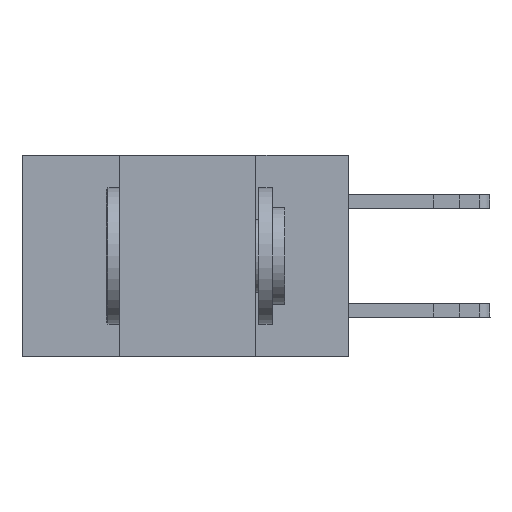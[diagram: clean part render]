
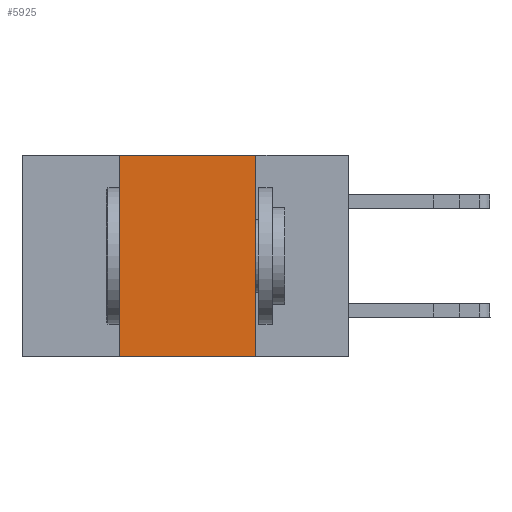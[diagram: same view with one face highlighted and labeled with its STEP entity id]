
A CAD part, left-side view. The second image highlights one B-rep face of the part: STEP entity #5925.
In plain terms, the highlighted planar face has unit normal (-1, 0, 0).
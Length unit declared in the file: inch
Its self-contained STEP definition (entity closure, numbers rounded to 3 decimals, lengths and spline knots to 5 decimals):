
#301 = EDGE_CURVE ( 'NONE', #20832, #16281, #1749, .T. ) ;
#938 = CARTESIAN_POINT ( 'NONE',  ( 0., 0.42, 0. ) ) ;
#1749 = LINE ( 'NONE', #8231, #21693 ) ;
#1785 = CARTESIAN_POINT ( 'NONE',  ( 0., 0.17, -0.37 ) ) ;
#4315 = EDGE_LOOP ( 'NONE', ( #10729, #6747, #22701, #14371 ) ) ;
#4501 = LINE ( 'NONE', #19665, #14265 ) ;
#4786 = DIRECTION ( 'NONE',  ( 0., -1., 0. ) ) ;
#5606 = VECTOR ( 'NONE', #4786, 39.37008 ) ;
#5701 = CARTESIAN_POINT ( 'NONE',  ( 0., 0.17, 0. ) ) ;
#5925 = ADVANCED_FACE ( 'NONE', ( #23440 ), #15261, .F. ) ;
#6152 = DIRECTION ( 'NONE',  ( 0., -1., 0. ) ) ;
#6747 = ORIENTED_EDGE ( 'NONE', *, *, #301, .F. ) ;
#7492 = DIRECTION ( 'NONE',  ( 1., 0., 0. ) ) ;
#8231 = CARTESIAN_POINT ( 'NONE',  ( 0., 0.6, 0. ) ) ;
#9570 = AXIS2_PLACEMENT_3D ( 'NONE', #19139, #7492, #20990 ) ;
#10049 = DIRECTION ( 'NONE',  ( 0., 0., -1. ) ) ;
#10248 = LINE ( 'NONE', #938, #24282 ) ;
#10729 = ORIENTED_EDGE ( 'NONE', *, *, #20351, .F. ) ;
#14265 = VECTOR ( 'NONE', #10049, 39.37008 ) ;
#14371 = ORIENTED_EDGE ( 'NONE', *, *, #22855, .T. ) ;
#15261 = PLANE ( 'NONE',  #9570 ) ;
#15355 = LINE ( 'NONE', #18387, #5606 ) ;
#15941 = CARTESIAN_POINT ( 'NONE',  ( 0., 0.42, 0. ) ) ;
#16281 = VERTEX_POINT ( 'NONE', #5701 ) ;
#18387 = CARTESIAN_POINT ( 'NONE',  ( 0., 0.6, -0.37 ) ) ;
#19139 = CARTESIAN_POINT ( 'NONE',  ( 0., 0.6, 0. ) ) ;
#19665 = CARTESIAN_POINT ( 'NONE',  ( 0., 0.17, 0. ) ) ;
#20351 = EDGE_CURVE ( 'NONE', #16281, #23147, #4501, .T. ) ;
#20446 = VERTEX_POINT ( 'NONE', #23723 ) ;
#20832 = VERTEX_POINT ( 'NONE', #15941 ) ;
#20990 = DIRECTION ( 'NONE',  ( 0., 0., -1. ) ) ;
#21592 = EDGE_CURVE ( 'NONE', #20446, #20832, #10248, .T. ) ;
#21693 = VECTOR ( 'NONE', #6152, 39.37008 ) ;
#22127 = DIRECTION ( 'NONE',  ( 0., 0., 1. ) ) ;
#22701 = ORIENTED_EDGE ( 'NONE', *, *, #21592, .F. ) ;
#22855 = EDGE_CURVE ( 'NONE', #20446, #23147, #15355, .T. ) ;
#23147 = VERTEX_POINT ( 'NONE', #1785 ) ;
#23440 = FACE_OUTER_BOUND ( 'NONE', #4315, .T. ) ;
#23723 = CARTESIAN_POINT ( 'NONE',  ( 0., 0.42, -0.37 ) ) ;
#24282 = VECTOR ( 'NONE', #22127, 39.37008 ) ;
